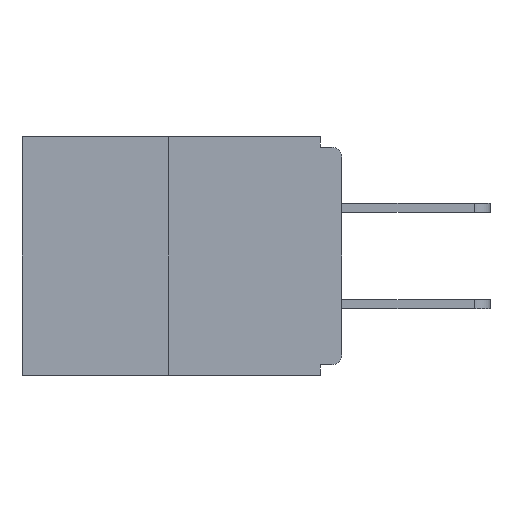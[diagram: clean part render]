
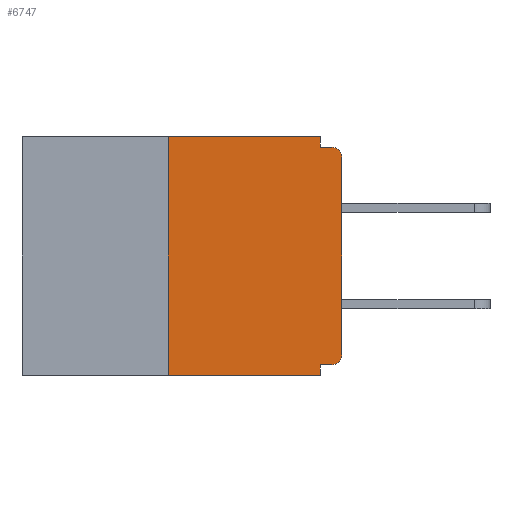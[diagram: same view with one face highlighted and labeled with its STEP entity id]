
A CAD part, left-side view. The second image highlights one B-rep face of the part: STEP entity #6747.
In plain terms, the highlighted planar face has unit normal (-1, 0, 0).
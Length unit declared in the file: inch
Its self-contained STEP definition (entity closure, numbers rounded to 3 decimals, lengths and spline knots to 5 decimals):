
#71 = VECTOR ( 'NONE', #13906, 39.37008 ) ;
#402 = EDGE_CURVE ( 'NONE', #12785, #4124, #8415, .T. ) ;
#444 = DIRECTION ( 'NONE',  ( 0., -1., 0. ) ) ;
#651 = EDGE_CURVE ( 'NONE', #4471, #7528, #10123, .T. ) ;
#703 = VECTOR ( 'NONE', #5098, 39.37008 ) ;
#1400 = ORIENTED_EDGE ( 'NONE', *, *, #402, .F. ) ;
#1412 = ORIENTED_EDGE ( 'NONE', *, *, #6795, .F. ) ;
#1422 = VECTOR ( 'NONE', #15732, 39.37008 ) ;
#1525 = ORIENTED_EDGE ( 'NONE', *, *, #5552, .F. ) ;
#1565 = DIRECTION ( 'NONE',  ( 0., 1., 0. ) ) ;
#1581 = VECTOR ( 'NONE', #12604, 39.37008 ) ;
#1619 = EDGE_CURVE ( 'NONE', #11439, #6116, #2385, .T. ) ;
#1763 = VECTOR ( 'NONE', #10811, 39.37008 ) ;
#1843 = CARTESIAN_POINT ( 'NONE',  ( 0., 0.015, -0.313 ) ) ;
#2385 = LINE ( 'NONE', #3855, #703 ) ;
#2516 = VERTEX_POINT ( 'NONE', #7189 ) ;
#3152 = CARTESIAN_POINT ( 'NONE',  ( 0., 0., -0.015 ) ) ;
#3561 = DIRECTION ( 'NONE',  ( -1., 0., 0. ) ) ;
#3718 = VECTOR ( 'NONE', #444, 39.37008 ) ;
#3855 = CARTESIAN_POINT ( 'NONE',  ( 0., 0., 0. ) ) ;
#3889 = PLANE ( 'NONE',  #14075 ) ;
#4046 = AXIS2_PLACEMENT_3D ( 'NONE', #5053, #3561, #6254 ) ;
#4124 = VERTEX_POINT ( 'NONE', #15869 ) ;
#4308 = CARTESIAN_POINT ( 'NONE',  ( 0., 0.46, 0. ) ) ;
#4320 = EDGE_CURVE ( 'NONE', #6116, #4124, #8685, .T. ) ;
#4471 = VERTEX_POINT ( 'NONE', #14911 ) ;
#4606 = DIRECTION ( 'NONE',  ( 0., 0., -1. ) ) ;
#5053 = CARTESIAN_POINT ( 'NONE',  ( 0., 0.015, -0.03 ) ) ;
#5098 = DIRECTION ( 'NONE',  ( 0., 0., 1. ) ) ;
#5469 = ORIENTED_EDGE ( 'NONE', *, *, #1619, .T. ) ;
#5552 = EDGE_CURVE ( 'NONE', #2516, #12785, #6483, .T. ) ;
#5857 = VECTOR ( 'NONE', #1565, 39.37008 ) ;
#6116 = VERTEX_POINT ( 'NONE', #14797 ) ;
#6152 = ORIENTED_EDGE ( 'NONE', *, *, #9787, .T. ) ;
#6230 = CARTESIAN_POINT ( 'NONE',  ( 0., 0.46, -0.343 ) ) ;
#6254 = DIRECTION ( 'NONE',  ( 0., 0., -1. ) ) ;
#6466 = VERTEX_POINT ( 'NONE', #15010 ) ;
#6483 = LINE ( 'NONE', #16565, #71 ) ;
#6747 = ADVANCED_FACE ( 'NONE', ( #10528 ), #3889, .F. ) ;
#6795 = EDGE_CURVE ( 'NONE', #12307, #6466, #9044, .T. ) ;
#6936 = CARTESIAN_POINT ( 'NONE',  ( 0., 0.031, -0.328 ) ) ;
#7189 = CARTESIAN_POINT ( 'NONE',  ( 0., 0.031, 0. ) ) ;
#7238 = CARTESIAN_POINT ( 'NONE',  ( 0., 0.25, -0.343 ) ) ;
#7502 = ORIENTED_EDGE ( 'NONE', *, *, #4320, .T. ) ;
#7528 = VERTEX_POINT ( 'NONE', #6936 ) ;
#8145 = EDGE_LOOP ( 'NONE', ( #9867, #1412, #6152, #12844, #12806, #10981, #5469, #7502, #1400, #1525 ) ) ;
#8415 = LINE ( 'NONE', #3152, #3718 ) ;
#8685 = CIRCLE ( 'NONE', #4046, 0.015 ) ;
#8826 = CARTESIAN_POINT ( 'NONE',  ( 0., 0.031, -0.343 ) ) ;
#9044 = LINE ( 'NONE', #11954, #1763 ) ;
#9261 = DIRECTION ( 'NONE',  ( 0., 0., -1. ) ) ;
#9450 = CARTESIAN_POINT ( 'NONE',  ( 0., 0., -0.313 ) ) ;
#9787 = EDGE_CURVE ( 'NONE', #12307, #17696, #10425, .T. ) ;
#9867 = ORIENTED_EDGE ( 'NONE', *, *, #14522, .F. ) ;
#9994 = CARTESIAN_POINT ( 'NONE',  ( 0., 0.031, -0.343 ) ) ;
#10123 = LINE ( 'NONE', #11111, #5857 ) ;
#10215 = EDGE_CURVE ( 'NONE', #4471, #11439, #16520, .T. ) ;
#10425 = LINE ( 'NONE', #6230, #1422 ) ;
#10528 = FACE_OUTER_BOUND ( 'NONE', #8145, .T. ) ;
#10811 = DIRECTION ( 'NONE',  ( 0., 0., 1. ) ) ;
#10981 = ORIENTED_EDGE ( 'NONE', *, *, #10215, .T. ) ;
#11111 = CARTESIAN_POINT ( 'NONE',  ( 0., 0., -0.328 ) ) ;
#11439 = VERTEX_POINT ( 'NONE', #9450 ) ;
#11491 = DIRECTION ( 'NONE',  ( 0., 0., -1. ) ) ;
#11719 = VECTOR ( 'NONE', #11491, 39.37008 ) ;
#11925 = LINE ( 'NONE', #9994, #11719 ) ;
#11954 = CARTESIAN_POINT ( 'NONE',  ( 0., 0.25, 0. ) ) ;
#12307 = VERTEX_POINT ( 'NONE', #7238 ) ;
#12564 = EDGE_CURVE ( 'NONE', #7528, #17696, #11925, .T. ) ;
#12604 = DIRECTION ( 'NONE',  ( 0., -1., 0. ) ) ;
#12785 = VERTEX_POINT ( 'NONE', #16483 ) ;
#12806 = ORIENTED_EDGE ( 'NONE', *, *, #651, .F. ) ;
#12844 = ORIENTED_EDGE ( 'NONE', *, *, #12564, .F. ) ;
#12947 = LINE ( 'NONE', #4308, #1581 ) ;
#13438 = AXIS2_PLACEMENT_3D ( 'NONE', #1843, #14280, #4606 ) ;
#13460 = DIRECTION ( 'NONE',  ( 1., 0., 0. ) ) ;
#13906 = DIRECTION ( 'NONE',  ( 0., 0., -1. ) ) ;
#14075 = AXIS2_PLACEMENT_3D ( 'NONE', #14826, #13460, #9261 ) ;
#14280 = DIRECTION ( 'NONE',  ( -1., 0., 0. ) ) ;
#14522 = EDGE_CURVE ( 'NONE', #6466, #2516, #12947, .T. ) ;
#14797 = CARTESIAN_POINT ( 'NONE',  ( 0., 0., -0.03 ) ) ;
#14826 = CARTESIAN_POINT ( 'NONE',  ( 0., 0.46, 0. ) ) ;
#14911 = CARTESIAN_POINT ( 'NONE',  ( 0., 0.015, -0.328 ) ) ;
#15010 = CARTESIAN_POINT ( 'NONE',  ( 0., 0.25, 0. ) ) ;
#15732 = DIRECTION ( 'NONE',  ( 0., -1., 0. ) ) ;
#15869 = CARTESIAN_POINT ( 'NONE',  ( 0., 0.015, -0.015 ) ) ;
#16483 = CARTESIAN_POINT ( 'NONE',  ( 0., 0.031, -0.015 ) ) ;
#16520 = CIRCLE ( 'NONE', #13438, 0.015 ) ;
#16565 = CARTESIAN_POINT ( 'NONE',  ( 0., 0.031, 0. ) ) ;
#17696 = VERTEX_POINT ( 'NONE', #8826 ) ;
